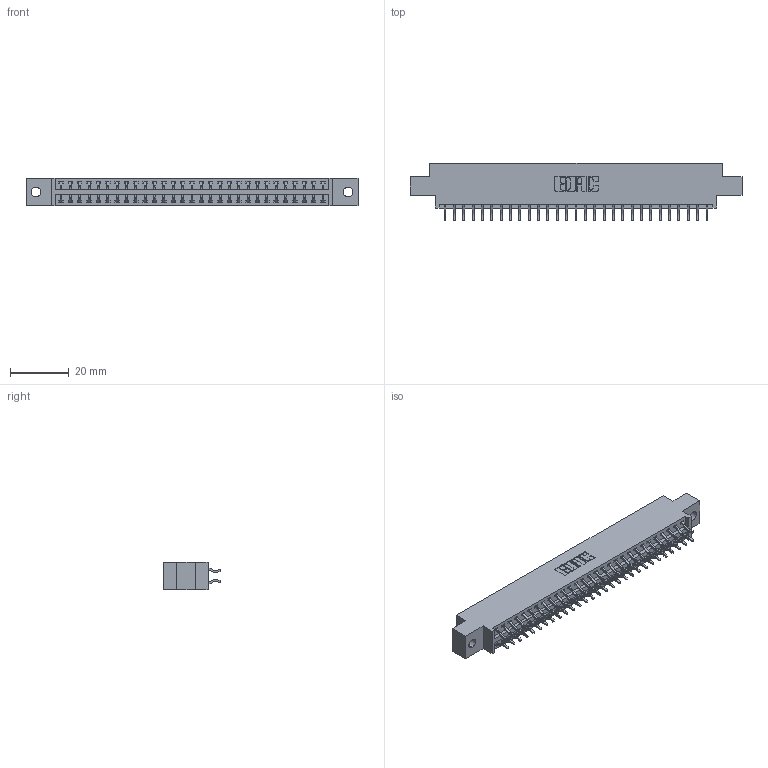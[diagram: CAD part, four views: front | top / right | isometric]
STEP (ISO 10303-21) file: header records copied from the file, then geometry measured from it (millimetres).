
FILE_DESCRIPTION (( 'STEP AP203' ), '1' );
FILE_NAME ('346-058-556-802.STEP', '2022-05-21T09:12:17', ( '' ), ( '' ), 'SwSTEP 2.0', 'SolidWorks 2020', '' );
FILE_SCHEMA (( 'CONFIG_CONTROL_DESIGN' ));
Length unit declared in the file: inch
Products named in the file (3): 346 Part_0.170 Offset - 0.128 Dia; 345-292-001_556 Tail; 346-058-556-802
Assembly tree (59 placements, depth 2):
  346-058-556-802
    346 Part_0.170 Offset - 0.128 Dia
    345-292-001_556 Tail  x58
Bounding box: 112.65 x 19.57 x 9.4 mm (x, y, z)
Volume: 10690.1 mm3; surface area: 14346.4 mm2
Topology: 59 solids, 59 shells, 3490 faces, 10375 edges, 6838 vertices
Faces by surface type: plane 2342, cylinder 1148
Entity records: 21031 total; most frequent: CARTESIAN_POINT 3500, ORIENTED_EDGE 3422, DIRECTION 3123, EDGE_CURVE 1711, LINE 1455, VECTOR 1455, VERTEX_POINT 1138, AXIS2_PLACEMENT_3D 834
